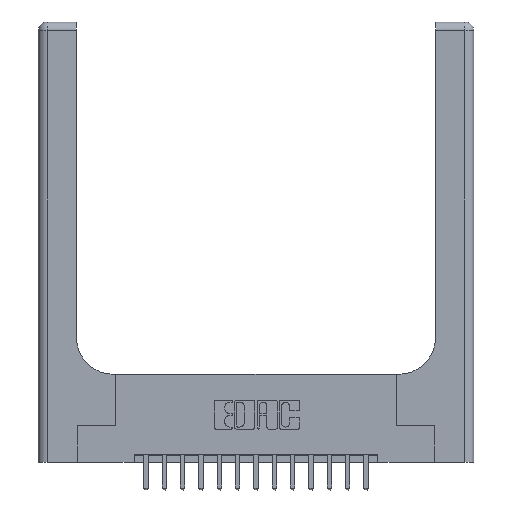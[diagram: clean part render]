
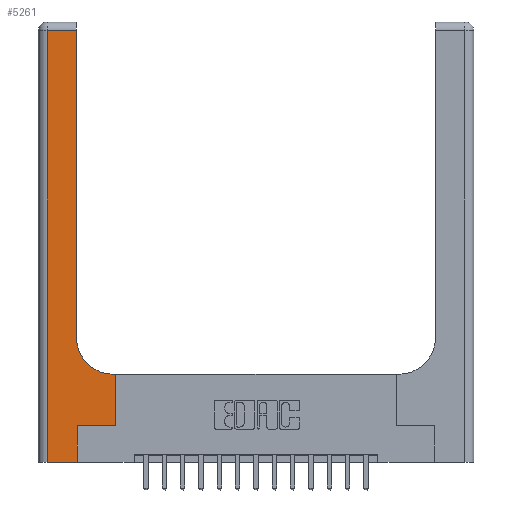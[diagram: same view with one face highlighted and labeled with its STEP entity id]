
A CAD part, top view. The second image highlights one B-rep face of the part: STEP entity #5261.
In plain terms, the highlighted planar face has unit normal (0, 0, 1).
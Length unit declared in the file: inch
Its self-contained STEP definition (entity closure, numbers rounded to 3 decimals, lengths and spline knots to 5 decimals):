
#142 = CARTESIAN_POINT ( 'NONE',  ( 0., 3., 0.37 ) ) ;
#179 = VECTOR ( 'NONE', #7942, 39.37008 ) ;
#303 = DIRECTION ( 'NONE',  ( 0., 1., 0. ) ) ;
#813 = VECTOR ( 'NONE', #303, 39.37008 ) ;
#963 = VERTEX_POINT ( 'NONE', #6975 ) ;
#1093 = DIRECTION ( 'NONE',  ( 1., 0., 0. ) ) ;
#1123 = VECTOR ( 'NONE', #1093, 39.37008 ) ;
#1150 = FACE_OUTER_BOUND ( 'NONE', #5009, .T. ) ;
#1222 = VERTEX_POINT ( 'NONE', #5167 ) ;
#1334 = CARTESIAN_POINT ( 'NONE',  ( 0.265, 0.25, 0.37 ) ) ;
#1656 = CARTESIAN_POINT ( 'NONE',  ( 0.265, 0., 0.37 ) ) ;
#1809 = DIRECTION ( 'NONE',  ( -1., 0., 0. ) ) ;
#2083 = CARTESIAN_POINT ( 'NONE',  ( 0.26, 0.6, 0.37 ) ) ;
#2589 = DIRECTION ( 'NONE',  ( 0., 1., 0. ) ) ;
#2695 = LINE ( 'NONE', #1334, #179 ) ;
#2773 = VERTEX_POINT ( 'NONE', #14484 ) ;
#2788 = ORIENTED_EDGE ( 'NONE', *, *, #11927, .T. ) ;
#2943 = LINE ( 'NONE', #1656, #813 ) ;
#3044 = EDGE_CURVE ( 'NONE', #12457, #13424, #12128, .T. ) ;
#3444 = LINE ( 'NONE', #10523, #9622 ) ;
#3493 = ORIENTED_EDGE ( 'NONE', *, *, #13216, .T. ) ;
#3608 = DIRECTION ( 'NONE',  ( 0., -1., 0. ) ) ;
#3714 = ORIENTED_EDGE ( 'NONE', *, *, #4359, .T. ) ;
#4016 = ORIENTED_EDGE ( 'NONE', *, *, #11148, .T. ) ;
#4230 = AXIS2_PLACEMENT_3D ( 'NONE', #17402, #10433, #16055 ) ;
#4359 = EDGE_CURVE ( 'NONE', #13424, #10371, #6838, .T. ) ;
#5009 = EDGE_LOOP ( 'NONE', ( #3714, #11484, #15802, #3493, #2788, #11580, #4016, #13870, #8827 ) ) ;
#5167 = CARTESIAN_POINT ( 'NONE',  ( 0.265, 0., 0.37 ) ) ;
#5261 = ADVANCED_FACE ( 'NONE', ( #1150 ), #5634, .F. ) ;
#5346 = EDGE_CURVE ( 'NONE', #2773, #12457, #6245, .T. ) ;
#5368 = DIRECTION ( 'NONE',  ( 0., 0., -1. ) ) ;
#5408 = LINE ( 'NONE', #6621, #1123 ) ;
#5634 = PLANE ( 'NONE',  #15604 ) ;
#6132 = VECTOR ( 'NONE', #2589, 39.37008 ) ;
#6185 = VERTEX_POINT ( 'NONE', #17185 ) ;
#6245 = LINE ( 'NONE', #2083, #16204 ) ;
#6409 = EDGE_CURVE ( 'NONE', #10371, #7285, #3444, .T. ) ;
#6581 = LINE ( 'NONE', #9703, #6132 ) ;
#6621 = CARTESIAN_POINT ( 'NONE',  ( 0., 0., 0.37 ) ) ;
#6838 = LINE ( 'NONE', #12515, #7930 ) ;
#6975 = CARTESIAN_POINT ( 'NONE',  ( 0.265, 0.25, 0.37 ) ) ;
#7285 = VERTEX_POINT ( 'NONE', #13655 ) ;
#7930 = VECTOR ( 'NONE', #17922, 39.37008 ) ;
#7942 = DIRECTION ( 'NONE',  ( 1., 0., 0. ) ) ;
#8249 = CARTESIAN_POINT ( 'NONE',  ( 0.51, 0.6, 0.37 ) ) ;
#8694 = CARTESIAN_POINT ( 'NONE',  ( 0.26, 0.85, 0.37 ) ) ;
#8827 = ORIENTED_EDGE ( 'NONE', *, *, #3044, .T. ) ;
#9066 = DIRECTION ( 'NONE',  ( -1., 0., 0. ) ) ;
#9267 = EDGE_CURVE ( 'NONE', #963, #10338, #2695, .T. ) ;
#9600 = LINE ( 'NONE', #15183, #12120 ) ;
#9622 = VECTOR ( 'NONE', #9066, 39.37008 ) ;
#9703 = CARTESIAN_POINT ( 'NONE',  ( 0.528, 0.25, 0.37 ) ) ;
#10338 = VERTEX_POINT ( 'NONE', #14154 ) ;
#10371 = VERTEX_POINT ( 'NONE', #13905 ) ;
#10433 = DIRECTION ( 'NONE',  ( 0., 0., -1. ) ) ;
#10523 = CARTESIAN_POINT ( 'NONE',  ( 0., 2.94, 0.37 ) ) ;
#10979 = DIRECTION ( 'NONE',  ( -1., 0., 0. ) ) ;
#11148 = EDGE_CURVE ( 'NONE', #10338, #2773, #6581, .T. ) ;
#11484 = ORIENTED_EDGE ( 'NONE', *, *, #6409, .T. ) ;
#11580 = ORIENTED_EDGE ( 'NONE', *, *, #9267, .T. ) ;
#11927 = EDGE_CURVE ( 'NONE', #1222, #963, #2943, .T. ) ;
#12120 = VECTOR ( 'NONE', #3608, 39.37008 ) ;
#12128 = CIRCLE ( 'NONE', #4230, 0.25 ) ;
#12457 = VERTEX_POINT ( 'NONE', #8249 ) ;
#12515 = CARTESIAN_POINT ( 'NONE',  ( 0.26, 3., 0.37 ) ) ;
#13216 = EDGE_CURVE ( 'NONE', #6185, #1222, #5408, .T. ) ;
#13424 = VERTEX_POINT ( 'NONE', #8694 ) ;
#13655 = CARTESIAN_POINT ( 'NONE',  ( 0.06, 2.94, 0.37 ) ) ;
#13870 = ORIENTED_EDGE ( 'NONE', *, *, #5346, .T. ) ;
#13905 = CARTESIAN_POINT ( 'NONE',  ( 0.26, 2.94, 0.37 ) ) ;
#14134 = EDGE_CURVE ( 'NONE', #7285, #6185, #9600, .T. ) ;
#14154 = CARTESIAN_POINT ( 'NONE',  ( 0.528, 0.25, 0.37 ) ) ;
#14484 = CARTESIAN_POINT ( 'NONE',  ( 0.528, 0.6, 0.37 ) ) ;
#15183 = CARTESIAN_POINT ( 'NONE',  ( 0.06, 3., 0.37 ) ) ;
#15604 = AXIS2_PLACEMENT_3D ( 'NONE', #142, #5368, #10979 ) ;
#15802 = ORIENTED_EDGE ( 'NONE', *, *, #14134, .T. ) ;
#16055 = DIRECTION ( 'NONE',  ( 1., 0., 0. ) ) ;
#16204 = VECTOR ( 'NONE', #1809, 39.37008 ) ;
#17185 = CARTESIAN_POINT ( 'NONE',  ( 0.06, 0., 0.37 ) ) ;
#17402 = CARTESIAN_POINT ( 'NONE',  ( 0.51, 0.85, 0.37 ) ) ;
#17922 = DIRECTION ( 'NONE',  ( 0., 1., 0. ) ) ;
